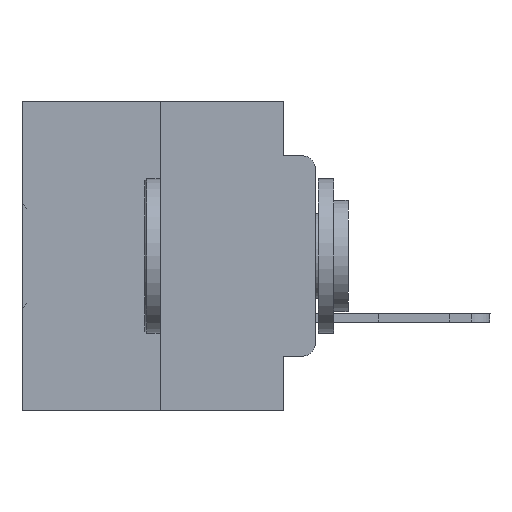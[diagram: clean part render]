
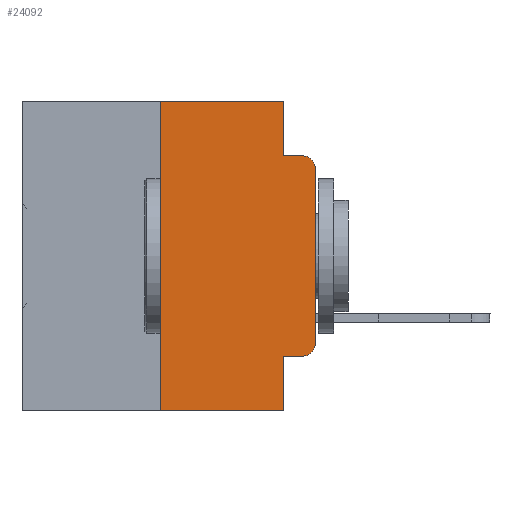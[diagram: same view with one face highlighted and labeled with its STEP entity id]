
A CAD part, left-side view. The second image highlights one B-rep face of the part: STEP entity #24092.
In plain terms, the highlighted planar face has unit normal (-1, 0, 0).
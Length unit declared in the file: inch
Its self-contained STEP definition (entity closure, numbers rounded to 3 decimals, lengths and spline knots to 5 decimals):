
#66 = CARTESIAN_POINT ( 'NONE',  ( 0., 0.02, -0.3915 ) ) ;
#237 = DIRECTION ( 'NONE',  ( -1., 0., 0. ) ) ;
#981 = CARTESIAN_POINT ( 'NONE',  ( 0., 0., -0.3915 ) ) ;
#1000 = VERTEX_POINT ( 'NONE', #31536 ) ;
#1775 = EDGE_CURVE ( 'NONE', #33345, #1000, #23522, .T. ) ;
#1862 = CARTESIAN_POINT ( 'NONE',  ( 0., 0.051, -0.0885 ) ) ;
#2707 = EDGE_CURVE ( 'NONE', #8618, #14207, #21763, .T. ) ;
#3244 = DIRECTION ( 'NONE',  ( 0., -1., 0. ) ) ;
#3360 = AXIS2_PLACEMENT_3D ( 'NONE', #23673, #34430, #12897 ) ;
#3425 = LINE ( 'NONE', #13997, #13898 ) ;
#3523 = VECTOR ( 'NONE', #33492, 39.37008 ) ;
#3565 = CARTESIAN_POINT ( 'NONE',  ( 0., 0.051, -0.0885 ) ) ;
#5222 = VERTEX_POINT ( 'NONE', #23771 ) ;
#5408 = ORIENTED_EDGE ( 'NONE', *, *, #12960, .F. ) ;
#6159 = LINE ( 'NONE', #12155, #3523 ) ;
#6364 = LINE ( 'NONE', #14322, #16674 ) ;
#7444 = FACE_OUTER_BOUND ( 'NONE', #20572, .T. ) ;
#7446 = EDGE_CURVE ( 'NONE', #22670, #16075, #28240, .T. ) ;
#8422 = CARTESIAN_POINT ( 'NONE',  ( 0., 0.02, -0.1085 ) ) ;
#8618 = VERTEX_POINT ( 'NONE', #12967 ) ;
#8893 = DIRECTION ( 'NONE',  ( 0., 0., -1. ) ) ;
#9127 = VERTEX_POINT ( 'NONE', #16216 ) ;
#10109 = DIRECTION ( 'NONE',  ( 0., -1., 0. ) ) ;
#10597 = ORIENTED_EDGE ( 'NONE', *, *, #28818, .T. ) ;
#10761 = LINE ( 'NONE', #22037, #26657 ) ;
#11410 = DIRECTION ( 'NONE',  ( 0., 0., -1. ) ) ;
#11534 = CARTESIAN_POINT ( 'NONE',  ( 0., 0.051, 0. ) ) ;
#11946 = VECTOR ( 'NONE', #10109, 39.37008 ) ;
#12129 = EDGE_CURVE ( 'NONE', #8618, #22670, #24503, .T. ) ;
#12155 = CARTESIAN_POINT ( 'NONE',  ( 0., 0.473, -0.5 ) ) ;
#12269 = ORIENTED_EDGE ( 'NONE', *, *, #19511, .T. ) ;
#12897 = DIRECTION ( 'NONE',  ( 0., 0., -1. ) ) ;
#12960 = EDGE_CURVE ( 'NONE', #5222, #9127, #3425, .T. ) ;
#12967 = CARTESIAN_POINT ( 'NONE',  ( 0., 0.051, -0.4115 ) ) ;
#13585 = DIRECTION ( 'NONE',  ( 0., -1., 0. ) ) ;
#13898 = VECTOR ( 'NONE', #3244, 39.37008 ) ;
#13997 = CARTESIAN_POINT ( 'NONE',  ( 0., 0.473, 0. ) ) ;
#14158 = CARTESIAN_POINT ( 'NONE',  ( 0., 0.02, -0.4115 ) ) ;
#14207 = VERTEX_POINT ( 'NONE', #23591 ) ;
#14322 = CARTESIAN_POINT ( 'NONE',  ( 0., 0., 0. ) ) ;
#16075 = VERTEX_POINT ( 'NONE', #981 ) ;
#16216 = CARTESIAN_POINT ( 'NONE',  ( 0., 0.051, 0. ) ) ;
#16382 = ORIENTED_EDGE ( 'NONE', *, *, #7446, .T. ) ;
#16423 = VERTEX_POINT ( 'NONE', #33480 ) ;
#16674 = VECTOR ( 'NONE', #24893, 39.37008 ) ;
#18009 = CARTESIAN_POINT ( 'NONE',  ( 0., 0., -0.1085 ) ) ;
#18628 = ORIENTED_EDGE ( 'NONE', *, *, #12129, .T. ) ;
#18992 = DIRECTION ( 'NONE',  ( -1., 0., 0. ) ) ;
#19511 = EDGE_CURVE ( 'NONE', #16075, #21526, #6364, .T. ) ;
#20572 = EDGE_LOOP ( 'NONE', ( #12269, #23107, #27746, #22055, #5408, #20806, #10597, #31053, #18628, #16382 ) ) ;
#20806 = ORIENTED_EDGE ( 'NONE', *, *, #29872, .F. ) ;
#20866 = VECTOR ( 'NONE', #8893, 39.37008 ) ;
#21420 = CARTESIAN_POINT ( 'NONE',  ( 0., 0.051, 0. ) ) ;
#21515 = DIRECTION ( 'NONE',  ( 0., 0., 1. ) ) ;
#21526 = VERTEX_POINT ( 'NONE', #18009 ) ;
#21552 = DIRECTION ( 'NONE',  ( 0., 0., -1. ) ) ;
#21582 = EDGE_CURVE ( 'NONE', #21526, #1000, #27967, .T. ) ;
#21763 = LINE ( 'NONE', #21420, #31973 ) ;
#22037 = CARTESIAN_POINT ( 'NONE',  ( 0., 0.25, 0. ) ) ;
#22055 = ORIENTED_EDGE ( 'NONE', *, *, #26358, .F. ) ;
#22670 = VERTEX_POINT ( 'NONE', #14158 ) ;
#23107 = ORIENTED_EDGE ( 'NONE', *, *, #21582, .T. ) ;
#23522 = LINE ( 'NONE', #1862, #11946 ) ;
#23591 = CARTESIAN_POINT ( 'NONE',  ( 0., 0.051, -0.5 ) ) ;
#23673 = CARTESIAN_POINT ( 'NONE',  ( 0., 0.473, 0. ) ) ;
#23771 = CARTESIAN_POINT ( 'NONE',  ( 0., 0.25, 0. ) ) ;
#24092 = ADVANCED_FACE ( 'NONE', ( #7444 ), #28947, .F. ) ;
#24503 = LINE ( 'NONE', #26803, #27915 ) ;
#24893 = DIRECTION ( 'NONE',  ( 0., 0., 1. ) ) ;
#24936 = LINE ( 'NONE', #11534, #20866 ) ;
#25141 = AXIS2_PLACEMENT_3D ( 'NONE', #8422, #18992, #11410 ) ;
#25417 = AXIS2_PLACEMENT_3D ( 'NONE', #66, #237, #21552 ) ;
#26358 = EDGE_CURVE ( 'NONE', #9127, #33345, #24936, .T. ) ;
#26657 = VECTOR ( 'NONE', #21515, 39.37008 ) ;
#26803 = CARTESIAN_POINT ( 'NONE',  ( 0., 0.051, -0.4115 ) ) ;
#27056 = DIRECTION ( 'NONE',  ( 0., 0., -1. ) ) ;
#27746 = ORIENTED_EDGE ( 'NONE', *, *, #1775, .F. ) ;
#27915 = VECTOR ( 'NONE', #13585, 39.37008 ) ;
#27967 = CIRCLE ( 'NONE', #25141, 0.02 ) ;
#28240 = CIRCLE ( 'NONE', #25417, 0.02 ) ;
#28818 = EDGE_CURVE ( 'NONE', #16423, #14207, #6159, .T. ) ;
#28947 = PLANE ( 'NONE',  #3360 ) ;
#29872 = EDGE_CURVE ( 'NONE', #16423, #5222, #10761, .T. ) ;
#31053 = ORIENTED_EDGE ( 'NONE', *, *, #2707, .F. ) ;
#31536 = CARTESIAN_POINT ( 'NONE',  ( 0., 0.02, -0.0885 ) ) ;
#31973 = VECTOR ( 'NONE', #27056, 39.37008 ) ;
#33345 = VERTEX_POINT ( 'NONE', #3565 ) ;
#33480 = CARTESIAN_POINT ( 'NONE',  ( 0., 0.25, -0.5 ) ) ;
#33492 = DIRECTION ( 'NONE',  ( 0., -1., 0. ) ) ;
#34430 = DIRECTION ( 'NONE',  ( 1., 0., 0. ) ) ;
